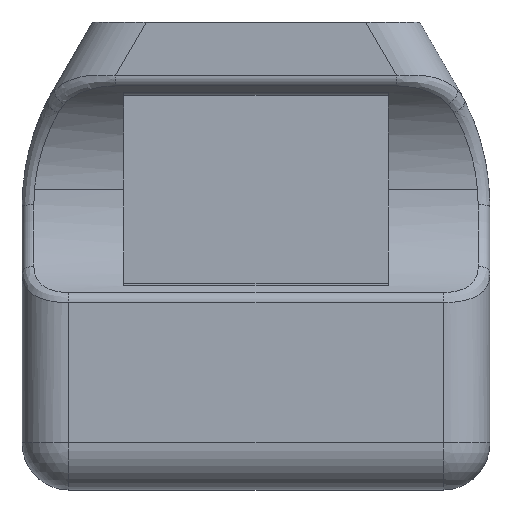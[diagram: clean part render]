
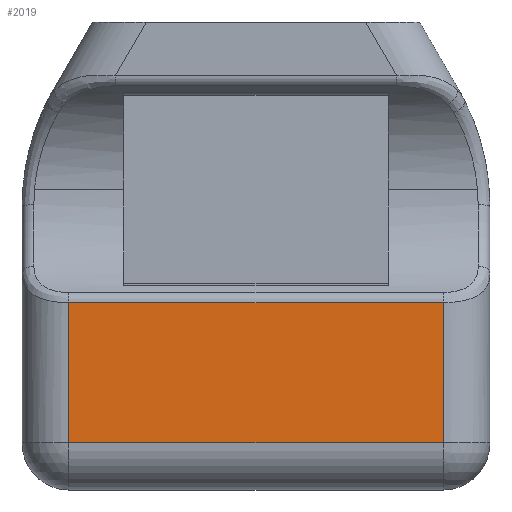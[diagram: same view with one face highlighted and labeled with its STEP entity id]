
A CAD part, top view. The second image highlights one B-rep face of the part: STEP entity #2019.
In plain terms, the highlighted face is planar.
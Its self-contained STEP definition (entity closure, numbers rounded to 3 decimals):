
#75 = PLANE ( 'NONE',  #673 ) ;
#112 = CARTESIAN_POINT ( 'NONE',  ( -8., -4.15, 3. ) ) ;
#255 = EDGE_CURVE ( 'NONE', #1910, #319, #2123, .T. ) ;
#279 = DIRECTION ( 'NONE',  ( 0., 1., 0. ) ) ;
#319 = VERTEX_POINT ( 'NONE', #2112 ) ;
#361 = ORIENTED_EDGE ( 'NONE', *, *, #651, .T. ) ;
#401 = CARTESIAN_POINT ( 'NONE',  ( 8., -4.15, -2.996 ) ) ;
#510 = CARTESIAN_POINT ( 'NONE',  ( -8., -4.15, -2.996 ) ) ;
#651 = EDGE_CURVE ( 'NONE', #319, #2130, #1307, .T. ) ;
#669 = ORIENTED_EDGE ( 'NONE', *, *, #1335, .T. ) ;
#673 = AXIS2_PLACEMENT_3D ( 'NONE', #1188, #279, #1747 ) ;
#683 = EDGE_LOOP ( 'NONE', ( #669, #1043, #1577, #361 ) ) ;
#702 = CARTESIAN_POINT ( 'NONE',  ( 10., -4.15, -2.996 ) ) ;
#875 = EDGE_CURVE ( 'NONE', #2086, #1910, #1587, .T. ) ;
#927 = CARTESIAN_POINT ( 'NONE',  ( -10., -4.15, 3. ) ) ;
#983 = VECTOR ( 'NONE', #1832, 1000. ) ;
#1043 = ORIENTED_EDGE ( 'NONE', *, *, #875, .T. ) ;
#1132 = VECTOR ( 'NONE', #1239, 1000. ) ;
#1173 = DIRECTION ( 'NONE',  ( 0., 0., 1. ) ) ;
#1188 = CARTESIAN_POINT ( 'NONE',  ( 10., -4.15, -15. ) ) ;
#1239 = DIRECTION ( 'NONE',  ( 1., 0., 0. ) ) ;
#1272 = CARTESIAN_POINT ( 'NONE',  ( -8., -4.15, -15. ) ) ;
#1301 = LINE ( 'NONE', #1272, #983 ) ;
#1307 = LINE ( 'NONE', #927, #2217 ) ;
#1335 = EDGE_CURVE ( 'NONE', #2130, #2086, #1301, .T. ) ;
#1577 = ORIENTED_EDGE ( 'NONE', *, *, #255, .T. ) ;
#1587 = LINE ( 'NONE', #702, #1132 ) ;
#1645 = VECTOR ( 'NONE', #1173, 1000. ) ;
#1657 = DIRECTION ( 'NONE',  ( -1., 0., 0. ) ) ;
#1747 = DIRECTION ( 'NONE',  ( 1., 0., 0. ) ) ;
#1832 = DIRECTION ( 'NONE',  ( 0., 0., -1. ) ) ;
#1910 = VERTEX_POINT ( 'NONE', #401 ) ;
#1947 = CARTESIAN_POINT ( 'NONE',  ( 8., -4.15, -15. ) ) ;
#2019 = ADVANCED_FACE ( 'NONE', ( #2082 ), #75, .F. ) ;
#2082 = FACE_OUTER_BOUND ( 'NONE', #683, .T. ) ;
#2086 = VERTEX_POINT ( 'NONE', #510 ) ;
#2112 = CARTESIAN_POINT ( 'NONE',  ( 8., -4.15, 3. ) ) ;
#2123 = LINE ( 'NONE', #1947, #1645 ) ;
#2130 = VERTEX_POINT ( 'NONE', #112 ) ;
#2217 = VECTOR ( 'NONE', #1657, 1000. ) ;
